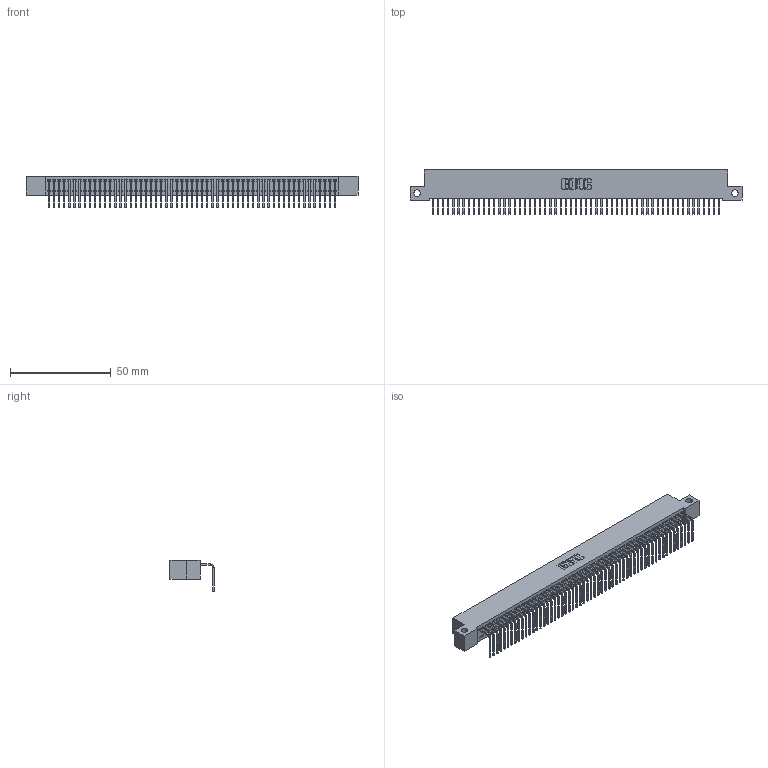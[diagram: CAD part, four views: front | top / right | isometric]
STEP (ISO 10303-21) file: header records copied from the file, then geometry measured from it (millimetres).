
FILE_DESCRIPTION (( 'STEP AP203' ), '1' );
FILE_NAME ('392-057-558-112.STEP', '2019-10-08T16:04:53', ( '' ), ( '' ), 'SwSTEP 2.0', 'SolidWorks 2016', '' );
FILE_SCHEMA (( 'CONFIG_CONTROL_DESIGN' ));
Length unit declared in the file: inch
Products named in the file (3): 342 Part_Side Mount; 345-292-001_558 Tail - 2; 392-057-558-112
Assembly tree (58 placements, depth 2):
  392-057-558-112
    342 Part_Side Mount
    345-292-001_558 Tail - 2  x57
Bounding box: 165.1 x 21.91 x 15.62 mm (x, y, z)
Volume: 14647.2 mm3; surface area: 22704.3 mm2
Topology: 58 solids, 58 shells, 3530 faces, 10673 edges, 7038 vertices
Faces by surface type: plane 2574, cylinder 956
Entity records: 32861 total; most frequent: CARTESIAN_POINT 5673, ORIENTED_EDGE 5666, DIRECTION 4755, EDGE_CURVE 2833, LINE 2705, VECTOR 2705, VERTEX_POINT 1886, AXIS2_PLACEMENT_3D 1025
